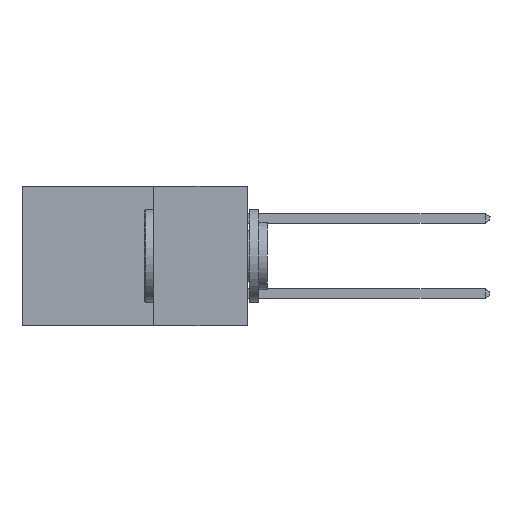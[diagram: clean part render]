
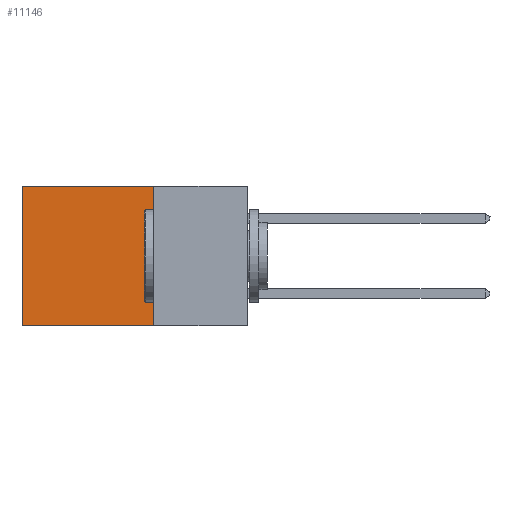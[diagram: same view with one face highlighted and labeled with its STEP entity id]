
A CAD part, left-side view. The second image highlights one B-rep face of the part: STEP entity #11146.
In plain terms, the highlighted planar face has unit normal (-1, 0, 0).
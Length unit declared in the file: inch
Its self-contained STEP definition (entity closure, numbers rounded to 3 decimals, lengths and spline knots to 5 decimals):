
#158 = EDGE_CURVE ( 'NONE', #9749, #7384, #19995, .T. ) ;
#866 = CARTESIAN_POINT ( 'NONE',  ( 0.298, 0.6, 0. ) ) ;
#1212 = CARTESIAN_POINT ( 'NONE',  ( 0.298, 0.25, 0. ) ) ;
#1493 = PLANE ( 'NONE',  #13006 ) ;
#3026 = EDGE_CURVE ( 'NONE', #4295, #17101, #8705, .T. ) ;
#4209 = EDGE_CURVE ( 'NONE', #4295, #9749, #9156, .T. ) ;
#4263 = VECTOR ( 'NONE', #7228, 39.37008 ) ;
#4295 = VERTEX_POINT ( 'NONE', #1212 ) ;
#4704 = VECTOR ( 'NONE', #19587, 39.37008 ) ;
#5296 = ORIENTED_EDGE ( 'NONE', *, *, #3026, .T. ) ;
#7123 = VECTOR ( 'NONE', #12563, 39.37008 ) ;
#7153 = LINE ( 'NONE', #14885, #15345 ) ;
#7228 = DIRECTION ( 'NONE',  ( 0., 1., 0. ) ) ;
#7247 = CARTESIAN_POINT ( 'NONE',  ( 0.298, 0.25, 0. ) ) ;
#7384 = VERTEX_POINT ( 'NONE', #8888 ) ;
#7437 = CARTESIAN_POINT ( 'NONE',  ( 0.298, 0.25, 0. ) ) ;
#8216 = DIRECTION ( 'NONE',  ( 1., 0., 0. ) ) ;
#8705 = LINE ( 'NONE', #7437, #4263 ) ;
#8888 = CARTESIAN_POINT ( 'NONE',  ( 0.298, 0.6, -0.37 ) ) ;
#9156 = LINE ( 'NONE', #7247, #4704 ) ;
#9749 = VERTEX_POINT ( 'NONE', #9923 ) ;
#9923 = CARTESIAN_POINT ( 'NONE',  ( 0.298, 0.25, -0.37 ) ) ;
#11146 = ADVANCED_FACE ( 'NONE', ( #14168 ), #1493, .F. ) ;
#11157 = ORIENTED_EDGE ( 'NONE', *, *, #14533, .T. ) ;
#11440 = ORIENTED_EDGE ( 'NONE', *, *, #4209, .F. ) ;
#12563 = DIRECTION ( 'NONE',  ( 0., 1., 0. ) ) ;
#12759 = EDGE_LOOP ( 'NONE', ( #11157, #19891, #11440, #5296 ) ) ;
#13006 = AXIS2_PLACEMENT_3D ( 'NONE', #17895, #8216, #19485 ) ;
#14168 = FACE_OUTER_BOUND ( 'NONE', #12759, .T. ) ;
#14533 = EDGE_CURVE ( 'NONE', #17101, #7384, #7153, .T. ) ;
#14885 = CARTESIAN_POINT ( 'NONE',  ( 0.298, 0.6, 0. ) ) ;
#15345 = VECTOR ( 'NONE', #16489, 39.37008 ) ;
#16489 = DIRECTION ( 'NONE',  ( 0., 0., -1. ) ) ;
#17101 = VERTEX_POINT ( 'NONE', #866 ) ;
#17895 = CARTESIAN_POINT ( 'NONE',  ( 0.298, 0.25, 0. ) ) ;
#19485 = DIRECTION ( 'NONE',  ( 0., 0., -1. ) ) ;
#19587 = DIRECTION ( 'NONE',  ( 0., 0., -1. ) ) ;
#19891 = ORIENTED_EDGE ( 'NONE', *, *, #158, .F. ) ;
#19995 = LINE ( 'NONE', #20639, #7123 ) ;
#20639 = CARTESIAN_POINT ( 'NONE',  ( 0.298, 0.25, -0.37 ) ) ;
